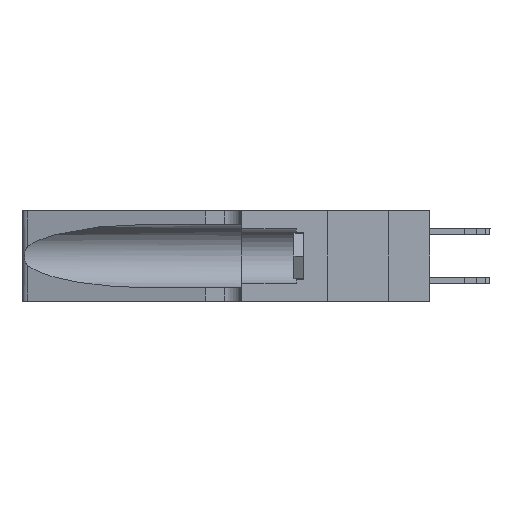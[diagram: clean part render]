
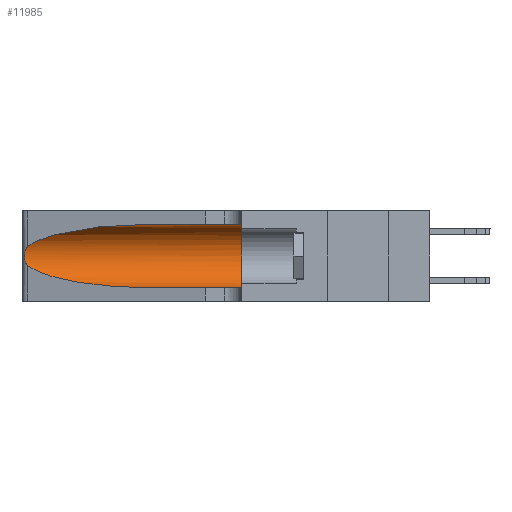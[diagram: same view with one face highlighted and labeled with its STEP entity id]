
A CAD part, left-side view. The second image highlights one B-rep face of the part: STEP entity #11985.
In plain terms, the highlighted cylindrical face has radius 3.308 mm (diameter 6.617 mm), a partial arc.
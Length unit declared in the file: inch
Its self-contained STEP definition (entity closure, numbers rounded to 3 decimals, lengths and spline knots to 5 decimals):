
#33 = DIRECTION ( 'NONE',  ( 0., 0., 1. ) ) ;
#1509 = CARTESIAN_POINT ( 'NONE',  ( 0.2373, 1.15595, 0.08982 ) ) ;
#1549 = CARTESIAN_POINT ( 'NONE',  ( 0.25487, 1.22718, 0.22369 ) ) ;
#1649 = VERTEX_POINT ( 'NONE', #1549 ) ;
#2522 = VECTOR ( 'NONE', #12289, 39.37008 ) ;
#3268 = CARTESIAN_POINT ( 'NONE',  ( 0.1305, 1.61858, 0.05475 ) ) ;
#3667 =( BOUNDED_CURVE ( )  B_SPLINE_CURVE ( 3, ( #13335, #6948, #4907, #21956 ),
 .UNSPECIFIED., .F., .F. ) 
 B_SPLINE_CURVE_WITH_KNOTS ( ( 4, 4 ),
 ( 1.5708, 2.84003 ),
 .UNSPECIFIED. ) 
 CURVE ( )  GEOMETRIC_REPRESENTATION_ITEM ( )  RATIONAL_B_SPLINE_CURVE ( ( 1., 0.87, 0.87, 1. ) ) 
 REPRESENTATION_ITEM ( '' )  );
#3721 = CARTESIAN_POINT ( 'NONE',  ( 0.25487, 1.22718, 0.14631 ) ) ;
#3810 = CARTESIAN_POINT ( 'NONE',  ( 0.25856, 1.23593, 0.16098 ) ) ;
#4907 = CARTESIAN_POINT ( 'NONE',  ( 0.2373, 1.15595, 0.28018 ) ) ;
#5365 = LINE ( 'NONE', #3268, #14627 ) ;
#6948 = CARTESIAN_POINT ( 'NONE',  ( 0.18966, 0.96281, 0.31525 ) ) ;
#6977 = CARTESIAN_POINT ( 'NONE',  ( 0.1305, 0.72297, 0.05475 ) ) ;
#7632 = EDGE_CURVE ( 'NONE', #18232, #11298, #11095, .T. ) ;
#8011 = CARTESIAN_POINT ( 'NONE',  ( 0.1305, 1.61858, 0.31525 ) ) ;
#8126 = CARTESIAN_POINT ( 'NONE',  ( 0.26075, 1.23896, 0.19203 ) ) ;
#8143 = FACE_OUTER_BOUND ( 'NONE', #16101, .T. ) ;
#10018 = CARTESIAN_POINT ( 'NONE',  ( 0.18966, 0.96281, 0.05475 ) ) ;
#10093 = CARTESIAN_POINT ( 'NONE',  ( 0.25487, 1.22718, 0.22369 ) ) ;
#10538 = EDGE_CURVE ( 'NONE', #19938, #25174, #5365, .T. ) ;
#10773 = EDGE_CURVE ( 'NONE', #1649, #18076, #19609, .T. ) ;
#11095 = LINE ( 'NONE', #8011, #2522 ) ;
#11298 = VERTEX_POINT ( 'NONE', #16648 ) ;
#11985 = ADVANCED_FACE ( 'NONE', ( #8143 ), #23732, .F. ) ;
#11991 = ORIENTED_EDGE ( 'NONE', *, *, #10773, .T. ) ;
#12128 = CARTESIAN_POINT ( 'NONE',  ( 0.26075, 1.23896, 0.178 ) ) ;
#12289 = DIRECTION ( 'NONE',  ( 0., -1., 0. ) ) ;
#12339 = DIRECTION ( 'NONE',  ( 0., -1., 0. ) ) ;
#12489 = CARTESIAN_POINT ( 'NONE',  ( 0.26018, 1.23835, 0.19895 ) ) ;
#13205 = ORIENTED_EDGE ( 'NONE', *, *, #24556, .T. ) ;
#13335 = CARTESIAN_POINT ( 'NONE',  ( 0.1305, 0.72297, 0.31525 ) ) ;
#13500 =( BOUNDED_CURVE ( )  B_SPLINE_CURVE ( 3, ( #26770, #1509, #10018, #20483 ),
 .UNSPECIFIED., .F., .F. ) 
 B_SPLINE_CURVE_WITH_KNOTS ( ( 4, 4 ),
 ( 3.44316, 4.71239 ),
 .UNSPECIFIED. ) 
 CURVE ( )  GEOMETRIC_REPRESENTATION_ITEM ( )  RATIONAL_B_SPLINE_CURVE ( ( 1., 0.87, 0.87, 1. ) ) 
 REPRESENTATION_ITEM ( '' )  );
#13572 = CARTESIAN_POINT ( 'NONE',  ( 0.1305, 0.35, 0.05475 ) ) ;
#14048 = ORIENTED_EDGE ( 'NONE', *, *, #10538, .T. ) ;
#14261 = CARTESIAN_POINT ( 'NONE',  ( 0.25555, 1.22993, 0.14849 ) ) ;
#14627 = VECTOR ( 'NONE', #16028, 39.37008 ) ;
#14730 = DIRECTION ( 'NONE',  ( 0., 1., 0. ) ) ;
#16028 = DIRECTION ( 'NONE',  ( 0., -1., 0. ) ) ;
#16101 = EDGE_LOOP ( 'NONE', ( #13205, #11991, #18187, #14048, #20888, #25857 ) ) ;
#16482 = CARTESIAN_POINT ( 'NONE',  ( 0.25787, 1.23484, 0.2124 ) ) ;
#16488 = CARTESIAN_POINT ( 'NONE',  ( 0.25487, 1.22718, 0.14631 ) ) ;
#16648 = CARTESIAN_POINT ( 'NONE',  ( 0.1305, 0.35, 0.31525 ) ) ;
#16680 = CARTESIAN_POINT ( 'NONE',  ( 0.1305, 0.72297, 0.31525 ) ) ;
#18076 = VERTEX_POINT ( 'NONE', #16488 ) ;
#18079 = EDGE_CURVE ( 'NONE', #18076, #19938, #13500, .T. ) ;
#18187 = ORIENTED_EDGE ( 'NONE', *, *, #18079, .T. ) ;
#18232 = VERTEX_POINT ( 'NONE', #16680 ) ;
#18251 = EDGE_CURVE ( 'NONE', #11298, #25174, #19701, .T. ) ;
#18512 = CARTESIAN_POINT ( 'NONE',  ( 0.25639, 1.23184, 0.21858 ) ) ;
#18816 = CARTESIAN_POINT ( 'NONE',  ( 0.1305, 1.61858, 0.185 ) ) ;
#19609 = B_SPLINE_CURVE_WITH_KNOTS ( 'NONE', 3,
 ( #10093, #20933, #18512, #16482, #24808, #12489, #8126, #12128, #27308, #3810, #26942, #22684, #14261, #3721 ),
 .UNSPECIFIED., .F., .F.,
 ( 4, 2, 2, 2, 2, 2, 4 ),
 ( 0., 0.00027, 0.00053, 0.00107, 0.0016, 0.00187, 0.00214 ),
 .UNSPECIFIED. ) ;
#19701 = CIRCLE ( 'NONE', #21965, 0.13025 ) ;
#19938 = VERTEX_POINT ( 'NONE', #6977 ) ;
#20483 = CARTESIAN_POINT ( 'NONE',  ( 0.1305, 0.72297, 0.05475 ) ) ;
#20888 = ORIENTED_EDGE ( 'NONE', *, *, #18251, .F. ) ;
#20933 = CARTESIAN_POINT ( 'NONE',  ( 0.25555, 1.22994, 0.2215 ) ) ;
#21956 = CARTESIAN_POINT ( 'NONE',  ( 0.25487, 1.22718, 0.22369 ) ) ;
#21965 = AXIS2_PLACEMENT_3D ( 'NONE', #23233, #14730, #33 ) ;
#22684 = CARTESIAN_POINT ( 'NONE',  ( 0.25639, 1.23186, 0.15144 ) ) ;
#22988 = DIRECTION ( 'NONE',  ( 0., 0., -1. ) ) ;
#23233 = CARTESIAN_POINT ( 'NONE',  ( 0.1305, 0.35, 0.185 ) ) ;
#23732 = CYLINDRICAL_SURFACE ( 'NONE', #25397, 0.13025 ) ;
#24556 = EDGE_CURVE ( 'NONE', #18232, #1649, #3667, .T. ) ;
#24808 = CARTESIAN_POINT ( 'NONE',  ( 0.25854, 1.2359, 0.20912 ) ) ;
#25174 = VERTEX_POINT ( 'NONE', #13572 ) ;
#25397 = AXIS2_PLACEMENT_3D ( 'NONE', #18816, #12339, #22988 ) ;
#25857 = ORIENTED_EDGE ( 'NONE', *, *, #7632, .F. ) ;
#26770 = CARTESIAN_POINT ( 'NONE',  ( 0.25487, 1.22718, 0.14631 ) ) ;
#26942 = CARTESIAN_POINT ( 'NONE',  ( 0.25789, 1.23486, 0.15765 ) ) ;
#27308 = CARTESIAN_POINT ( 'NONE',  ( 0.26017, 1.23833, 0.17102 ) ) ;
